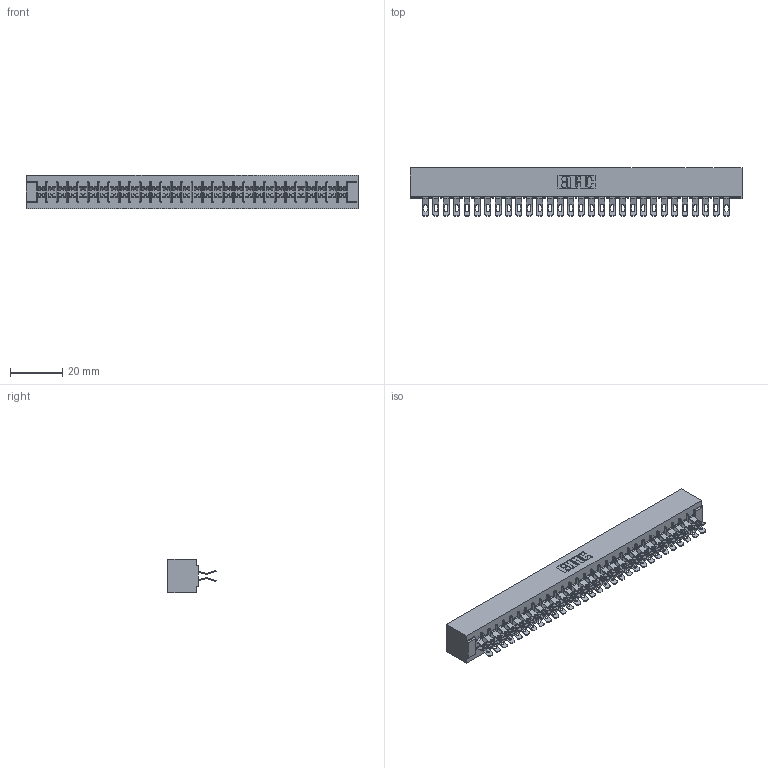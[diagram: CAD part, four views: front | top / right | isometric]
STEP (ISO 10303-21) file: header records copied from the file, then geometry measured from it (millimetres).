
FILE_DESCRIPTION (( 'STEP AP203' ), '1' );
FILE_NAME ('355-060-555-501.STEP', '2019-09-12T14:00:10', ( '' ), ( '' ), 'SwSTEP 2.0', 'SolidWorks 2016', '' );
FILE_SCHEMA (( 'CONFIG_CONTROL_DESIGN' ));
Length unit declared in the file: inch
Products named in the file (3): 305 Part_No Mounting; 355-060-555-501; 305-290-001_555
Assembly tree (61 placements, depth 2):
  355-060-555-501
    305 Part_No Mounting
    305-290-001_555  x60
Bounding box: 126.75 x 18.41 x 12.7 mm (x, y, z)
Volume: 13396.8 mm3; surface area: 18971.5 mm2
Topology: 61 solids, 61 shells, 4068 faces, 12142 edges, 7932 vertices
Faces by surface type: plane 1984, cylinder 1964, sphere 120
Entity records: 34289 total; most frequent: CARTESIAN_POINT 5690, ORIENTED_EDGE 5636, DIRECTION 5506, EDGE_CURVE 2818, VECTOR 2250, LINE 2250, VERTEX_POINT 1796, AXIS2_PLACEMENT_3D 1628
